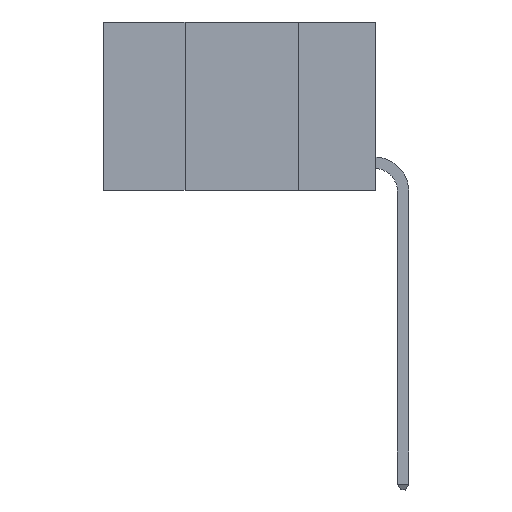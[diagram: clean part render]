
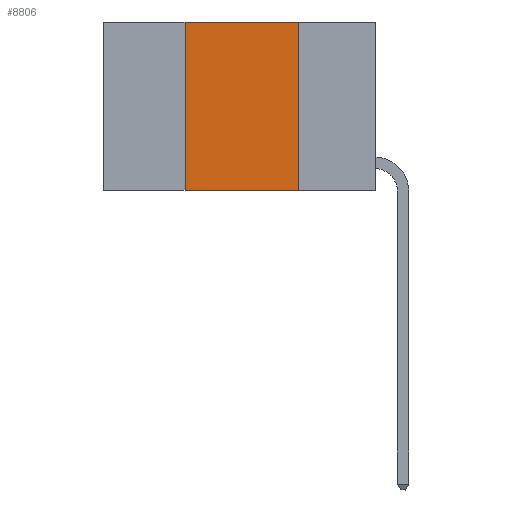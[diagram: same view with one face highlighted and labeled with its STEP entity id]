
A CAD part, left-side view. The second image highlights one B-rep face of the part: STEP entity #8806.
In plain terms, the highlighted planar face has unit normal (-1, 0, 0).
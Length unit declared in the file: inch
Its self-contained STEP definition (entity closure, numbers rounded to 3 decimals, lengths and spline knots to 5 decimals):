
#301 = DIRECTION ( 'NONE',  ( 0., -1., 0. ) ) ;
#316 = LINE ( 'NONE', #8336, #7729 ) ;
#764 = VERTEX_POINT ( 'NONE', #3497 ) ;
#782 = VECTOR ( 'NONE', #1810, 39.37008 ) ;
#928 = VERTEX_POINT ( 'NONE', #10917 ) ;
#967 = ORIENTED_EDGE ( 'NONE', *, *, #1733, .F. ) ;
#1558 = CARTESIAN_POINT ( 'NONE',  ( 0., 0.6, 0. ) ) ;
#1733 = EDGE_CURVE ( 'NONE', #764, #4076, #316, .T. ) ;
#1810 = DIRECTION ( 'NONE',  ( 0., 0., 1. ) ) ;
#1939 = DIRECTION ( 'NONE',  ( 0., -1., 0. ) ) ;
#2181 = ORIENTED_EDGE ( 'NONE', *, *, #3084, .F. ) ;
#2490 = VERTEX_POINT ( 'NONE', #10741 ) ;
#2878 = LINE ( 'NONE', #3886, #12750 ) ;
#3074 = EDGE_LOOP ( 'NONE', ( #2181, #967, #4120, #12500 ) ) ;
#3084 = EDGE_CURVE ( 'NONE', #4076, #928, #6446, .T. ) ;
#3102 = EDGE_CURVE ( 'NONE', #2490, #764, #8764, .T. ) ;
#3173 = EDGE_CURVE ( 'NONE', #2490, #928, #2878, .T. ) ;
#3497 = CARTESIAN_POINT ( 'NONE',  ( 0., 0.42, 0. ) ) ;
#3886 = CARTESIAN_POINT ( 'NONE',  ( 0., 0.6, -0.37 ) ) ;
#4076 = VERTEX_POINT ( 'NONE', #5835 ) ;
#4120 = ORIENTED_EDGE ( 'NONE', *, *, #3102, .F. ) ;
#5580 = DIRECTION ( 'NONE',  ( 0., 0., -1. ) ) ;
#5587 = FACE_OUTER_BOUND ( 'NONE', #3074, .T. ) ;
#5835 = CARTESIAN_POINT ( 'NONE',  ( 0., 0.17, 0. ) ) ;
#6446 = LINE ( 'NONE', #10678, #9070 ) ;
#6577 = AXIS2_PLACEMENT_3D ( 'NONE', #1558, #11485, #5580 ) ;
#7683 = DIRECTION ( 'NONE',  ( 0., 0., -1. ) ) ;
#7729 = VECTOR ( 'NONE', #301, 39.37008 ) ;
#8336 = CARTESIAN_POINT ( 'NONE',  ( 0., 0.6, 0. ) ) ;
#8499 = PLANE ( 'NONE',  #6577 ) ;
#8749 = CARTESIAN_POINT ( 'NONE',  ( 0., 0.42, 0. ) ) ;
#8764 = LINE ( 'NONE', #8749, #782 ) ;
#8806 = ADVANCED_FACE ( 'NONE', ( #5587 ), #8499, .F. ) ;
#9070 = VECTOR ( 'NONE', #7683, 39.37008 ) ;
#10678 = CARTESIAN_POINT ( 'NONE',  ( 0., 0.17, 0. ) ) ;
#10741 = CARTESIAN_POINT ( 'NONE',  ( 0., 0.42, -0.37 ) ) ;
#10917 = CARTESIAN_POINT ( 'NONE',  ( 0., 0.17, -0.37 ) ) ;
#11485 = DIRECTION ( 'NONE',  ( 1., 0., 0. ) ) ;
#12500 = ORIENTED_EDGE ( 'NONE', *, *, #3173, .T. ) ;
#12750 = VECTOR ( 'NONE', #1939, 39.37008 ) ;
